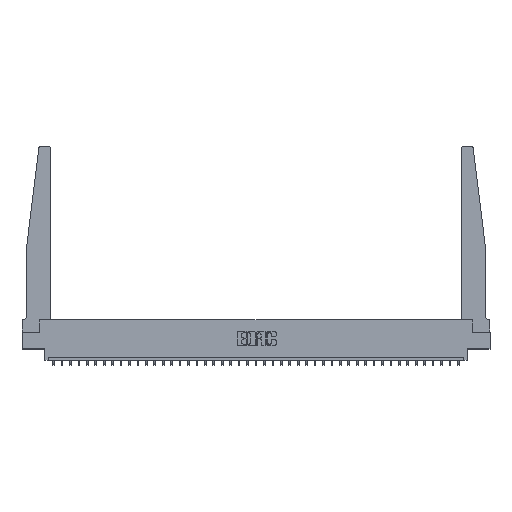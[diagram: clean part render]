
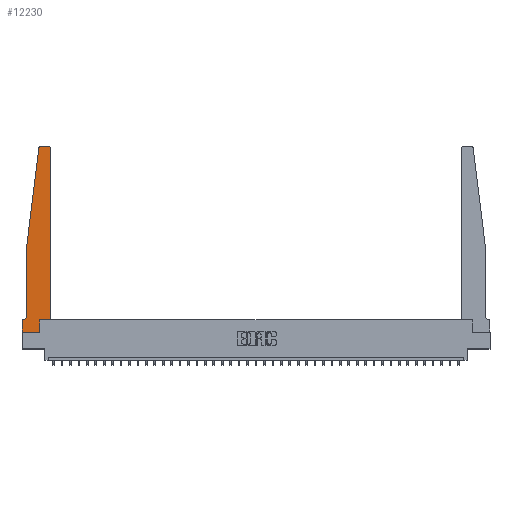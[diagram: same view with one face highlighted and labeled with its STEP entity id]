
A CAD part, top view. The second image highlights one B-rep face of the part: STEP entity #12230.
In plain terms, the highlighted planar face has unit normal (0, 0, 1).
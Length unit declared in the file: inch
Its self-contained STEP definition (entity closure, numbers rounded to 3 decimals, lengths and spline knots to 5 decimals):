
#151 = DIRECTION ( 'NONE',  ( 1., 0., 0. ) ) ;
#548 = CARTESIAN_POINT ( 'NONE',  ( 0.015, 0.1875, 0.37 ) ) ;
#563 = CARTESIAN_POINT ( 'NONE',  ( 0.425, 0.18, 0.37 ) ) ;
#590 = EDGE_CURVE ( 'NONE', #34867, #14418, #22248, .T. ) ;
#912 = AXIS2_PLACEMENT_3D ( 'NONE', #15825, #13352, #8066 ) ;
#1413 = DIRECTION ( 'NONE',  ( 0., 1., 0. ) ) ;
#1758 = CARTESIAN_POINT ( 'NONE',  ( 0.425, 0.18, 0.37 ) ) ;
#2098 = VECTOR ( 'NONE', #13755, 39.37008 ) ;
#2272 = ORIENTED_EDGE ( 'NONE', *, *, #17496, .T. ) ;
#2477 = CARTESIAN_POINT ( 'NONE',  ( 0.065, 0.1875, 0.37 ) ) ;
#2998 = CARTESIAN_POINT ( 'NONE',  ( 0.2605, 0.18, 0.37 ) ) ;
#4397 = DIRECTION ( 'NONE',  ( 1., 0., 0. ) ) ;
#4481 = FACE_OUTER_BOUND ( 'NONE', #10600, .T. ) ;
#4650 = CARTESIAN_POINT ( 'NONE',  ( 0., 0.1875, 0.37 ) ) ;
#4755 = DIRECTION ( 'NONE',  ( 0., 0., 1. ) ) ;
#6313 = VECTOR ( 'NONE', #30195, 39.37008 ) ;
#6527 = ORIENTED_EDGE ( 'NONE', *, *, #34278, .T. ) ;
#6719 = CARTESIAN_POINT ( 'NONE',  ( 0., 0., 0.37 ) ) ;
#7098 = ORIENTED_EDGE ( 'NONE', *, *, #34358, .T. ) ;
#7597 = LINE ( 'NONE', #26686, #23360 ) ;
#7674 = VERTEX_POINT ( 'NONE', #563 ) ;
#7997 = VECTOR ( 'NONE', #4397, 39.37008 ) ;
#8066 = DIRECTION ( 'NONE',  ( -1., 0., 0. ) ) ;
#8123 = VERTEX_POINT ( 'NONE', #19422 ) ;
#8699 = DIRECTION ( 'NONE',  ( 0., 0., 1. ) ) ;
#8853 = CARTESIAN_POINT ( 'NONE',  ( 0.065, 0.2375, 0.37 ) ) ;
#8910 = VERTEX_POINT ( 'NONE', #33416 ) ;
#9317 = CARTESIAN_POINT ( 'NONE',  ( 0., 0.1875, 0.37 ) ) ;
#9589 = EDGE_CURVE ( 'NONE', #15074, #14853, #7597, .T. ) ;
#9611 = ORIENTED_EDGE ( 'NONE', *, *, #24802, .T. ) ;
#9940 = PLANE ( 'NONE',  #14260 ) ;
#10600 = EDGE_LOOP ( 'NONE', ( #31217, #9611, #2272, #11769, #25308, #6527, #31457, #32207, #7098, #16013, #21828, #18644 ) ) ;
#11508 = DIRECTION ( 'NONE',  ( 1., 0., 0. ) ) ;
#11769 = ORIENTED_EDGE ( 'NONE', *, *, #33851, .T. ) ;
#11825 = CARTESIAN_POINT ( 'NONE',  ( 0.425, 2.72, 0.37 ) ) ;
#12230 = ADVANCED_FACE ( 'NONE', ( #4481 ), #9940, .T. ) ;
#12559 = LINE ( 'NONE', #18049, #20175 ) ;
#12735 = DIRECTION ( 'NONE',  ( -0.122, -0.992, 0. ) ) ;
#12871 = DIRECTION ( 'NONE',  ( 1., 0., 0. ) ) ;
#13136 = LINE ( 'NONE', #34849, #28573 ) ;
#13352 = DIRECTION ( 'NONE',  ( 0., 0., -1. ) ) ;
#13433 = VERTEX_POINT ( 'NONE', #11825 ) ;
#13569 = CARTESIAN_POINT ( 'NONE',  ( 0.2605, 0., 0.37 ) ) ;
#13755 = DIRECTION ( 'NONE',  ( 0., 1., 0. ) ) ;
#14260 = AXIS2_PLACEMENT_3D ( 'NONE', #4650, #20906, #23915 ) ;
#14418 = VERTEX_POINT ( 'NONE', #25855 ) ;
#14853 = VERTEX_POINT ( 'NONE', #6719 ) ;
#14926 = EDGE_CURVE ( 'NONE', #13433, #34867, #24588, .T. ) ;
#15074 = VERTEX_POINT ( 'NONE', #9317 ) ;
#15728 = VERTEX_POINT ( 'NONE', #8853 ) ;
#15785 = DIRECTION ( 'NONE',  ( 0., -1., 0. ) ) ;
#15825 = CARTESIAN_POINT ( 'NONE',  ( 0.015, 0.2375, 0.37 ) ) ;
#15849 = LINE ( 'NONE', #16203, #19318 ) ;
#16013 = ORIENTED_EDGE ( 'NONE', *, *, #27855, .T. ) ;
#16203 = CARTESIAN_POINT ( 'NONE',  ( 0., 0., 0.37 ) ) ;
#16965 = CARTESIAN_POINT ( 'NONE',  ( 0.425, 0.18, 0.37 ) ) ;
#17212 = AXIS2_PLACEMENT_3D ( 'NONE', #17838, #4755, #12871 ) ;
#17260 = VECTOR ( 'NONE', #1413, 39.37008 ) ;
#17266 = CIRCLE ( 'NONE', #912, 0.05 ) ;
#17335 = CARTESIAN_POINT ( 'NONE',  ( 0.27653, 2.72, 0.37 ) ) ;
#17496 = EDGE_CURVE ( 'NONE', #8910, #20355, #12559, .T. ) ;
#17757 = EDGE_CURVE ( 'NONE', #7674, #13433, #28447, .T. ) ;
#17838 = CARTESIAN_POINT ( 'NONE',  ( 0.395, 2.72, 0.37 ) ) ;
#18030 = VERTEX_POINT ( 'NONE', #13569 ) ;
#18049 = CARTESIAN_POINT ( 'NONE',  ( 0.065, 1.25, 0.37 ) ) ;
#18533 = LINE ( 'NONE', #2998, #2098 ) ;
#18644 = ORIENTED_EDGE ( 'NONE', *, *, #14926, .T. ) ;
#19318 = VECTOR ( 'NONE', #151, 39.37008 ) ;
#19422 = CARTESIAN_POINT ( 'NONE',  ( 0.2605, 0.18, 0.37 ) ) ;
#20175 = VECTOR ( 'NONE', #12735, 39.37008 ) ;
#20355 = VERTEX_POINT ( 'NONE', #29018 ) ;
#20906 = DIRECTION ( 'NONE',  ( 0., 0., 1. ) ) ;
#21726 = CARTESIAN_POINT ( 'NONE',  ( 0.25, 2.75, 0.37 ) ) ;
#21828 = ORIENTED_EDGE ( 'NONE', *, *, #17757, .T. ) ;
#22248 = LINE ( 'NONE', #21726, #6313 ) ;
#22613 = CIRCLE ( 'NONE', #29363, 0.03 ) ;
#23360 = VECTOR ( 'NONE', #26855, 39.37008 ) ;
#23915 = DIRECTION ( 'NONE',  ( 1., 0., 0. ) ) ;
#24588 = CIRCLE ( 'NONE', #17212, 0.03 ) ;
#24802 = EDGE_CURVE ( 'NONE', #14418, #8910, #22613, .T. ) ;
#25308 = ORIENTED_EDGE ( 'NONE', *, *, #33524, .T. ) ;
#25855 = CARTESIAN_POINT ( 'NONE',  ( 0.27653, 2.75, 0.37 ) ) ;
#26502 = DIRECTION ( 'NONE',  ( -1., 0., 0. ) ) ;
#26686 = CARTESIAN_POINT ( 'NONE',  ( 0., 0., 0.37 ) ) ;
#26795 = EDGE_CURVE ( 'NONE', #14853, #18030, #15849, .T. ) ;
#26855 = DIRECTION ( 'NONE',  ( 0., -1., 0. ) ) ;
#27855 = EDGE_CURVE ( 'NONE', #8123, #7674, #34394, .T. ) ;
#28447 = LINE ( 'NONE', #16965, #17260 ) ;
#28573 = VECTOR ( 'NONE', #15785, 39.37008 ) ;
#29018 = CARTESIAN_POINT ( 'NONE',  ( 0.065, 1.25, 0.37 ) ) ;
#29363 = AXIS2_PLACEMENT_3D ( 'NONE', #17335, #8699, #11508 ) ;
#29986 = CARTESIAN_POINT ( 'NONE',  ( 0.395, 2.75, 0.37 ) ) ;
#30195 = DIRECTION ( 'NONE',  ( -1., 0., 0. ) ) ;
#31217 = ORIENTED_EDGE ( 'NONE', *, *, #590, .T. ) ;
#31457 = ORIENTED_EDGE ( 'NONE', *, *, #9589, .T. ) ;
#31737 = VERTEX_POINT ( 'NONE', #548 ) ;
#32207 = ORIENTED_EDGE ( 'NONE', *, *, #26795, .T. ) ;
#32301 = LINE ( 'NONE', #2477, #34140 ) ;
#33416 = CARTESIAN_POINT ( 'NONE',  ( 0.24675, 2.72367, 0.37 ) ) ;
#33524 = EDGE_CURVE ( 'NONE', #15728, #31737, #17266, .T. ) ;
#33851 = EDGE_CURVE ( 'NONE', #20355, #15728, #13136, .T. ) ;
#34140 = VECTOR ( 'NONE', #26502, 39.37008 ) ;
#34278 = EDGE_CURVE ( 'NONE', #31737, #15074, #32301, .T. ) ;
#34358 = EDGE_CURVE ( 'NONE', #18030, #8123, #18533, .T. ) ;
#34394 = LINE ( 'NONE', #1758, #7997 ) ;
#34849 = CARTESIAN_POINT ( 'NONE',  ( 0.065, 1.25, 0.37 ) ) ;
#34867 = VERTEX_POINT ( 'NONE', #29986 ) ;
